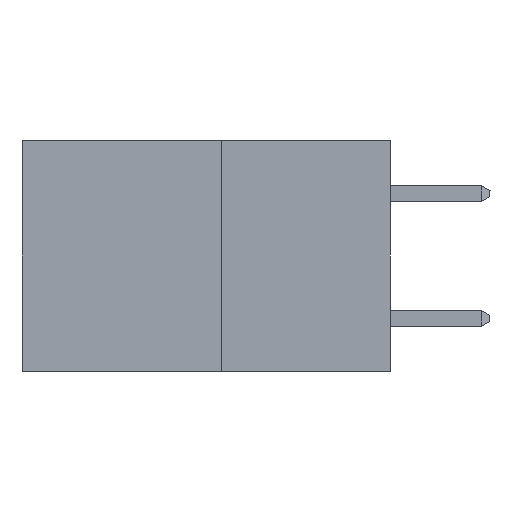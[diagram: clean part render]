
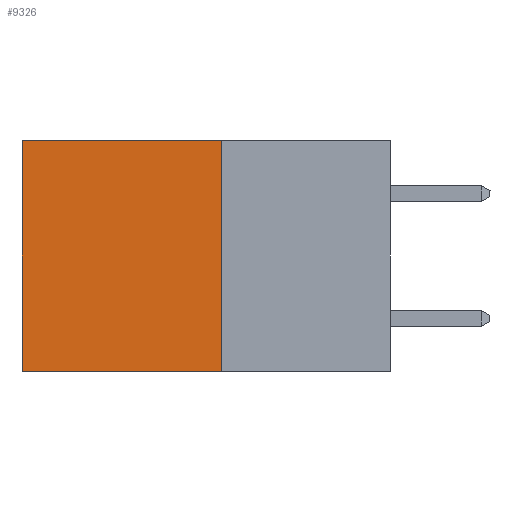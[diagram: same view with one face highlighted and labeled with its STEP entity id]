
A CAD part, left-side view. The second image highlights one B-rep face of the part: STEP entity #9326.
In plain terms, the highlighted planar face has unit normal (-1, 0, 0).
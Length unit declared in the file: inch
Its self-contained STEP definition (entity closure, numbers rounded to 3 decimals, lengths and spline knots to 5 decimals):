
#291 = EDGE_CURVE ( 'NONE', #4150, #5324, #6969, .T. ) ;
#626 = VECTOR ( 'NONE', #4130, 39.37008 ) ;
#790 = CARTESIAN_POINT ( 'NONE',  ( 0.277, 0.27, -0.37 ) ) ;
#1186 = CARTESIAN_POINT ( 'NONE',  ( 0.277, 0.27, -0.37 ) ) ;
#1288 = AXIS2_PLACEMENT_3D ( 'NONE', #6653, #4397, #9835 ) ;
#2010 = VECTOR ( 'NONE', #6040, 39.37008 ) ;
#2342 = EDGE_CURVE ( 'NONE', #6816, #4376, #6799, .T. ) ;
#2371 = EDGE_CURVE ( 'NONE', #5324, #4376, #4541, .T. ) ;
#2516 = VECTOR ( 'NONE', #9929, 39.37008 ) ;
#2694 = VECTOR ( 'NONE', #4955, 39.37008 ) ;
#3439 = ORIENTED_EDGE ( 'NONE', *, *, #2371, .F. ) ;
#3447 = EDGE_CURVE ( 'NONE', #4150, #6816, #6060, .T. ) ;
#4130 = DIRECTION ( 'NONE',  ( 0., 0., -1. ) ) ;
#4150 = VERTEX_POINT ( 'NONE', #6627 ) ;
#4376 = VERTEX_POINT ( 'NONE', #6857 ) ;
#4397 = DIRECTION ( 'NONE',  ( 1., 0., 0. ) ) ;
#4541 = LINE ( 'NONE', #790, #2516 ) ;
#4610 = CARTESIAN_POINT ( 'NONE',  ( 0.277, 0.59, 0. ) ) ;
#4955 = DIRECTION ( 'NONE',  ( 0., 0., -1. ) ) ;
#5324 = VERTEX_POINT ( 'NONE', #7362 ) ;
#5686 = FACE_OUTER_BOUND ( 'NONE', #5840, .T. ) ;
#5840 = EDGE_LOOP ( 'NONE', ( #9834, #3439, #7541, #10080 ) ) ;
#5949 = CARTESIAN_POINT ( 'NONE',  ( 0.277, 0.27, 0. ) ) ;
#6040 = DIRECTION ( 'NONE',  ( 0., 1., 0. ) ) ;
#6060 = LINE ( 'NONE', #5949, #2010 ) ;
#6627 = CARTESIAN_POINT ( 'NONE',  ( 0.277, 0.27, 0. ) ) ;
#6653 = CARTESIAN_POINT ( 'NONE',  ( 0.277, 0.27, -0.37 ) ) ;
#6799 = LINE ( 'NONE', #8142, #626 ) ;
#6816 = VERTEX_POINT ( 'NONE', #4610 ) ;
#6857 = CARTESIAN_POINT ( 'NONE',  ( 0.277, 0.59, -0.37 ) ) ;
#6969 = LINE ( 'NONE', #1186, #2694 ) ;
#7362 = CARTESIAN_POINT ( 'NONE',  ( 0.277, 0.27, -0.37 ) ) ;
#7541 = ORIENTED_EDGE ( 'NONE', *, *, #291, .F. ) ;
#8142 = CARTESIAN_POINT ( 'NONE',  ( 0.277, 0.59, -0.37 ) ) ;
#8293 = PLANE ( 'NONE',  #1288 ) ;
#9326 = ADVANCED_FACE ( 'NONE', ( #5686 ), #8293, .F. ) ;
#9834 = ORIENTED_EDGE ( 'NONE', *, *, #2342, .T. ) ;
#9835 = DIRECTION ( 'NONE',  ( 0., 0., -1. ) ) ;
#9929 = DIRECTION ( 'NONE',  ( 0., 1., 0. ) ) ;
#10080 = ORIENTED_EDGE ( 'NONE', *, *, #3447, .T. ) ;
